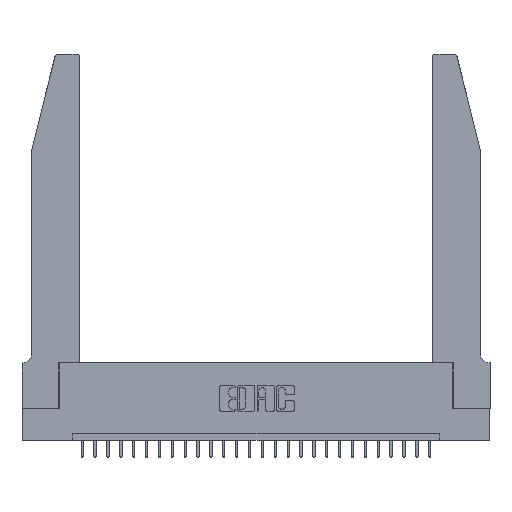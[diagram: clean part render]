
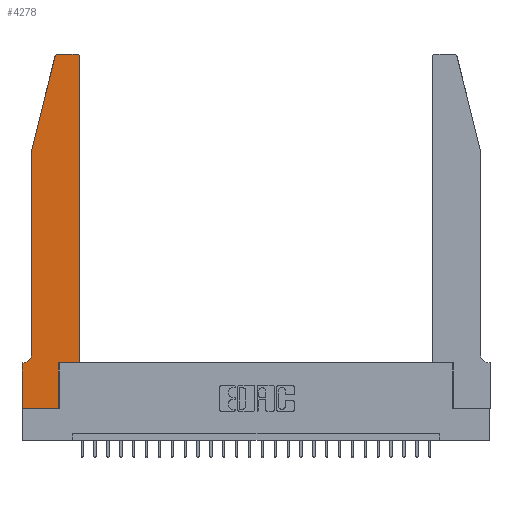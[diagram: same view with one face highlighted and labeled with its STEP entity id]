
A CAD part, top view. The second image highlights one B-rep face of the part: STEP entity #4278.
In plain terms, the highlighted planar face has unit normal (0, 0, 1).
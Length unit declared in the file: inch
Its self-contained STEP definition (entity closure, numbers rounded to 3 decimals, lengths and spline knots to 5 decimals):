
#142 = VERTEX_POINT ( 'NONE', #925 ) ;
#212 = CARTESIAN_POINT ( 'NONE',  ( 0., 0.35, 0.37 ) ) ;
#348 = EDGE_CURVE ( 'NONE', #25613, #142, #23438, .T. ) ;
#451 = VERTEX_POINT ( 'NONE', #21618 ) ;
#575 = EDGE_CURVE ( 'NONE', #4163, #26518, #2515, .T. ) ;
#925 = CARTESIAN_POINT ( 'NONE',  ( 0.284, 2.75, 0.37 ) ) ;
#1154 = LINE ( 'NONE', #9740, #22814 ) ;
#1992 = VERTEX_POINT ( 'NONE', #13375 ) ;
#2018 = CARTESIAN_POINT ( 'NONE',  ( 0., 0.35, 0.37 ) ) ;
#2257 = VERTEX_POINT ( 'NONE', #25587 ) ;
#2327 = LINE ( 'NONE', #15300, #11253 ) ;
#2515 = LINE ( 'NONE', #4373, #16406 ) ;
#3206 = EDGE_CURVE ( 'NONE', #26518, #13533, #6119, .T. ) ;
#3663 = VECTOR ( 'NONE', #8047, 39.37008 ) ;
#3873 = FACE_OUTER_BOUND ( 'NONE', #17926, .T. ) ;
#3927 = AXIS2_PLACEMENT_3D ( 'NONE', #2018, #16699, #25249 ) ;
#4163 = VERTEX_POINT ( 'NONE', #7241 ) ;
#4278 = ADVANCED_FACE ( 'NONE', ( #3873 ), #27213, .T. ) ;
#4373 = CARTESIAN_POINT ( 'NONE',  ( 0.0755, 0.35, 0.37 ) ) ;
#4605 = EDGE_CURVE ( 'NONE', #13533, #1992, #1154, .T. ) ;
#4954 = EDGE_CURVE ( 'NONE', #142, #15437, #14730, .T. ) ;
#5378 = ORIENTED_EDGE ( 'NONE', *, *, #22193, .T. ) ;
#5443 = VERTEX_POINT ( 'NONE', #21842 ) ;
#6014 = CARTESIAN_POINT ( 'NONE',  ( 0.2605, 2.75, 0.37 ) ) ;
#6119 = LINE ( 'NONE', #23274, #19401 ) ;
#6349 = AXIS2_PLACEMENT_3D ( 'NONE', #15577, #19532, #25974 ) ;
#6468 = ORIENTED_EDGE ( 'NONE', *, *, #575, .T. ) ;
#7241 = CARTESIAN_POINT ( 'NONE',  ( 0.0055, 0.35, 0.37 ) ) ;
#7463 = CARTESIAN_POINT ( 'NONE',  ( 0.4505, 0.35, 0.37 ) ) ;
#7596 = ORIENTED_EDGE ( 'NONE', *, *, #18400, .T. ) ;
#7720 = AXIS2_PLACEMENT_3D ( 'NONE', #7979, #16612, #22920 ) ;
#7979 = CARTESIAN_POINT ( 'NONE',  ( 0.0055, 0.42, 0.37 ) ) ;
#8047 = DIRECTION ( 'NONE',  ( -0.239, -0.971, 0. ) ) ;
#8250 = CARTESIAN_POINT ( 'NONE',  ( 0.284, 2.72, 0.37 ) ) ;
#8724 = CARTESIAN_POINT ( 'NONE',  ( 0.4205, 2.75, 0.37 ) ) ;
#9007 = CIRCLE ( 'NONE', #6349, 0.03 ) ;
#9649 = CARTESIAN_POINT ( 'NONE',  ( 0.0755, 2., 0.37 ) ) ;
#9740 = CARTESIAN_POINT ( 'NONE',  ( 0., 0., 0.37 ) ) ;
#9879 = LINE ( 'NONE', #24938, #3663 ) ;
#10449 = LINE ( 'NONE', #12996, #25758 ) ;
#10885 = EDGE_CURVE ( 'NONE', #1992, #5443, #2327, .T. ) ;
#11253 = VECTOR ( 'NONE', #15439, 39.37008 ) ;
#11416 = EDGE_CURVE ( 'NONE', #15437, #19712, #9879, .T. ) ;
#12996 = CARTESIAN_POINT ( 'NONE',  ( 0.4505, 0.35, 0.37 ) ) ;
#13235 = VECTOR ( 'NONE', #14800, 39.37008 ) ;
#13327 = ORIENTED_EDGE ( 'NONE', *, *, #4954, .T. ) ;
#13354 = EDGE_CURVE ( 'NONE', #5443, #25260, #10449, .T. ) ;
#13375 = CARTESIAN_POINT ( 'NONE',  ( 0.2865, 0., 0.37 ) ) ;
#13533 = VERTEX_POINT ( 'NONE', #26341 ) ;
#13567 = ORIENTED_EDGE ( 'NONE', *, *, #19430, .T. ) ;
#14730 = CIRCLE ( 'NONE', #24119, 0.03 ) ;
#14800 = DIRECTION ( 'NONE',  ( 0., 1., 0. ) ) ;
#15300 = CARTESIAN_POINT ( 'NONE',  ( 0.2865, 0.35, 0.37 ) ) ;
#15437 = VERTEX_POINT ( 'NONE', #18438 ) ;
#15439 = DIRECTION ( 'NONE',  ( 0., 1., 0. ) ) ;
#15577 = CARTESIAN_POINT ( 'NONE',  ( 0.4205, 2.72, 0.37 ) ) ;
#16361 = ORIENTED_EDGE ( 'NONE', *, *, #4605, .T. ) ;
#16406 = VECTOR ( 'NONE', #19985, 39.37008 ) ;
#16612 = DIRECTION ( 'NONE',  ( 0., 0., -1. ) ) ;
#16699 = DIRECTION ( 'NONE',  ( 0., 0., 1. ) ) ;
#17808 = DIRECTION ( 'NONE',  ( 1., 0., 0. ) ) ;
#17926 = EDGE_LOOP ( 'NONE', ( #19737, #13327, #22729, #23362, #13567, #6468, #19364, #16361, #23121, #22762, #5378, #7596 ) ) ;
#18052 = LINE ( 'NONE', #7463, #13235 ) ;
#18400 = EDGE_CURVE ( 'NONE', #451, #25613, #9007, .T. ) ;
#18438 = CARTESIAN_POINT ( 'NONE',  ( 0.25487, 2.72718, 0.37 ) ) ;
#18706 = DIRECTION ( 'NONE',  ( -1., 0., 0. ) ) ;
#19130 = DIRECTION ( 'NONE',  ( 1., 0., 0. ) ) ;
#19364 = ORIENTED_EDGE ( 'NONE', *, *, #3206, .T. ) ;
#19401 = VECTOR ( 'NONE', #25526, 39.37008 ) ;
#19430 = EDGE_CURVE ( 'NONE', #2257, #4163, #19865, .T. ) ;
#19532 = DIRECTION ( 'NONE',  ( 0., 0., 1. ) ) ;
#19712 = VERTEX_POINT ( 'NONE', #9649 ) ;
#19737 = ORIENTED_EDGE ( 'NONE', *, *, #348, .T. ) ;
#19865 = CIRCLE ( 'NONE', #7720, 0.07 ) ;
#19985 = DIRECTION ( 'NONE',  ( -1., 0., 0. ) ) ;
#20033 = VECTOR ( 'NONE', #18706, 39.37008 ) ;
#20384 = EDGE_CURVE ( 'NONE', #19712, #2257, #27046, .T. ) ;
#21258 = VECTOR ( 'NONE', #27182, 39.37008 ) ;
#21439 = DIRECTION ( 'NONE',  ( 1., 0., 0. ) ) ;
#21618 = CARTESIAN_POINT ( 'NONE',  ( 0.4505, 2.72, 0.37 ) ) ;
#21842 = CARTESIAN_POINT ( 'NONE',  ( 0.2865, 0.35, 0.37 ) ) ;
#22193 = EDGE_CURVE ( 'NONE', #25260, #451, #18052, .T. ) ;
#22561 = CARTESIAN_POINT ( 'NONE',  ( 0.0755, 2., 0.37 ) ) ;
#22729 = ORIENTED_EDGE ( 'NONE', *, *, #11416, .T. ) ;
#22762 = ORIENTED_EDGE ( 'NONE', *, *, #13354, .T. ) ;
#22814 = VECTOR ( 'NONE', #17808, 39.37008 ) ;
#22920 = DIRECTION ( 'NONE',  ( -1., 0., 0. ) ) ;
#23121 = ORIENTED_EDGE ( 'NONE', *, *, #10885, .T. ) ;
#23274 = CARTESIAN_POINT ( 'NONE',  ( 0., 0., 0.37 ) ) ;
#23362 = ORIENTED_EDGE ( 'NONE', *, *, #20384, .T. ) ;
#23438 = LINE ( 'NONE', #6014, #20033 ) ;
#24119 = AXIS2_PLACEMENT_3D ( 'NONE', #8250, #25293, #19130 ) ;
#24938 = CARTESIAN_POINT ( 'NONE',  ( 0.0755, 2., 0.37 ) ) ;
#25249 = DIRECTION ( 'NONE',  ( 1., 0., 0. ) ) ;
#25260 = VERTEX_POINT ( 'NONE', #25657 ) ;
#25293 = DIRECTION ( 'NONE',  ( 0., 0., 1. ) ) ;
#25526 = DIRECTION ( 'NONE',  ( 0., -1., 0. ) ) ;
#25587 = CARTESIAN_POINT ( 'NONE',  ( 0.0755, 0.42, 0.37 ) ) ;
#25613 = VERTEX_POINT ( 'NONE', #8724 ) ;
#25657 = CARTESIAN_POINT ( 'NONE',  ( 0.4505, 0.35, 0.37 ) ) ;
#25758 = VECTOR ( 'NONE', #21439, 39.37008 ) ;
#25974 = DIRECTION ( 'NONE',  ( 1., 0., 0. ) ) ;
#26341 = CARTESIAN_POINT ( 'NONE',  ( 0., 0., 0.37 ) ) ;
#26518 = VERTEX_POINT ( 'NONE', #212 ) ;
#27046 = LINE ( 'NONE', #22561, #21258 ) ;
#27182 = DIRECTION ( 'NONE',  ( 0., -1., 0. ) ) ;
#27213 = PLANE ( 'NONE',  #3927 ) ;
